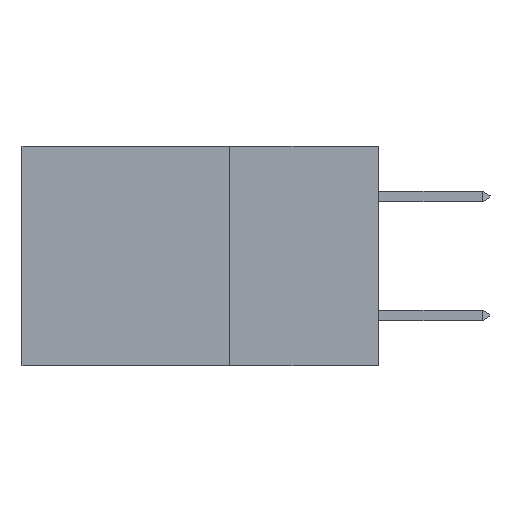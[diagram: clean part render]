
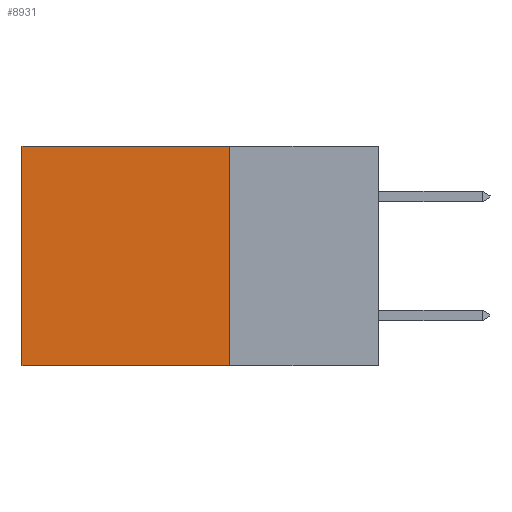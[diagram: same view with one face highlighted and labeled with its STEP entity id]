
A CAD part, left-side view. The second image highlights one B-rep face of the part: STEP entity #8931.
In plain terms, the highlighted planar face has unit normal (-1, 0, 0).
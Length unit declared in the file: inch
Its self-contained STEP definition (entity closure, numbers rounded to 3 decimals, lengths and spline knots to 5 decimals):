
#13 = VECTOR ( 'NONE', #11018, 39.37008 ) ;
#50 = DIRECTION ( 'NONE',  ( 1., 0., 0. ) ) ;
#268 = EDGE_LOOP ( 'NONE', ( #2883, #4294, #6910, #9288 ) ) ;
#752 = VERTEX_POINT ( 'NONE', #3293 ) ;
#1135 = PLANE ( 'NONE',  #15400 ) ;
#1337 = EDGE_CURVE ( 'NONE', #752, #4405, #16248, .T. ) ;
#2557 = LINE ( 'NONE', #3741, #17449 ) ;
#2883 = ORIENTED_EDGE ( 'NONE', *, *, #1337, .T. ) ;
#3293 = CARTESIAN_POINT ( 'NONE',  ( 0.2615, 0.6, 0. ) ) ;
#3741 = CARTESIAN_POINT ( 'NONE',  ( 0.2615, 0.25, 0. ) ) ;
#3838 = VECTOR ( 'NONE', #8662, 39.37008 ) ;
#4145 = EDGE_CURVE ( 'NONE', #17116, #4405, #15029, .T. ) ;
#4191 = VERTEX_POINT ( 'NONE', #9869 ) ;
#4294 = ORIENTED_EDGE ( 'NONE', *, *, #4145, .F. ) ;
#4400 = CARTESIAN_POINT ( 'NONE',  ( 0.2615, 0.6, -0.37 ) ) ;
#4405 = VERTEX_POINT ( 'NONE', #10429 ) ;
#4864 = DIRECTION ( 'NONE',  ( 0., 0., -1. ) ) ;
#5207 = DIRECTION ( 'NONE',  ( 0., 0., -1. ) ) ;
#6106 = CARTESIAN_POINT ( 'NONE',  ( 0.2615, 0.25, -0.37 ) ) ;
#6910 = ORIENTED_EDGE ( 'NONE', *, *, #7128, .F. ) ;
#6932 = CARTESIAN_POINT ( 'NONE',  ( 0.2615, 0.25, -0.37 ) ) ;
#7128 = EDGE_CURVE ( 'NONE', #4191, #17116, #15815, .T. ) ;
#8176 = FACE_OUTER_BOUND ( 'NONE', #268, .T. ) ;
#8662 = DIRECTION ( 'NONE',  ( 0., 0., -1. ) ) ;
#8931 = ADVANCED_FACE ( 'NONE', ( #8176 ), #1135, .F. ) ;
#9288 = ORIENTED_EDGE ( 'NONE', *, *, #10256, .T. ) ;
#9869 = CARTESIAN_POINT ( 'NONE',  ( 0.2615, 0.25, 0. ) ) ;
#10256 = EDGE_CURVE ( 'NONE', #4191, #752, #2557, .T. ) ;
#10429 = CARTESIAN_POINT ( 'NONE',  ( 0.2615, 0.6, -0.37 ) ) ;
#11018 = DIRECTION ( 'NONE',  ( 0., 1., 0. ) ) ;
#12151 = DIRECTION ( 'NONE',  ( 0., 1., 0. ) ) ;
#12199 = VECTOR ( 'NONE', #4864, 39.37008 ) ;
#14620 = CARTESIAN_POINT ( 'NONE',  ( 0.2615, 0.25, -0.37 ) ) ;
#15029 = LINE ( 'NONE', #6932, #13 ) ;
#15400 = AXIS2_PLACEMENT_3D ( 'NONE', #14620, #50, #5207 ) ;
#15815 = LINE ( 'NONE', #6106, #12199 ) ;
#16248 = LINE ( 'NONE', #4400, #3838 ) ;
#16259 = CARTESIAN_POINT ( 'NONE',  ( 0.2615, 0.25, -0.37 ) ) ;
#17116 = VERTEX_POINT ( 'NONE', #16259 ) ;
#17449 = VECTOR ( 'NONE', #12151, 39.37008 ) ;
